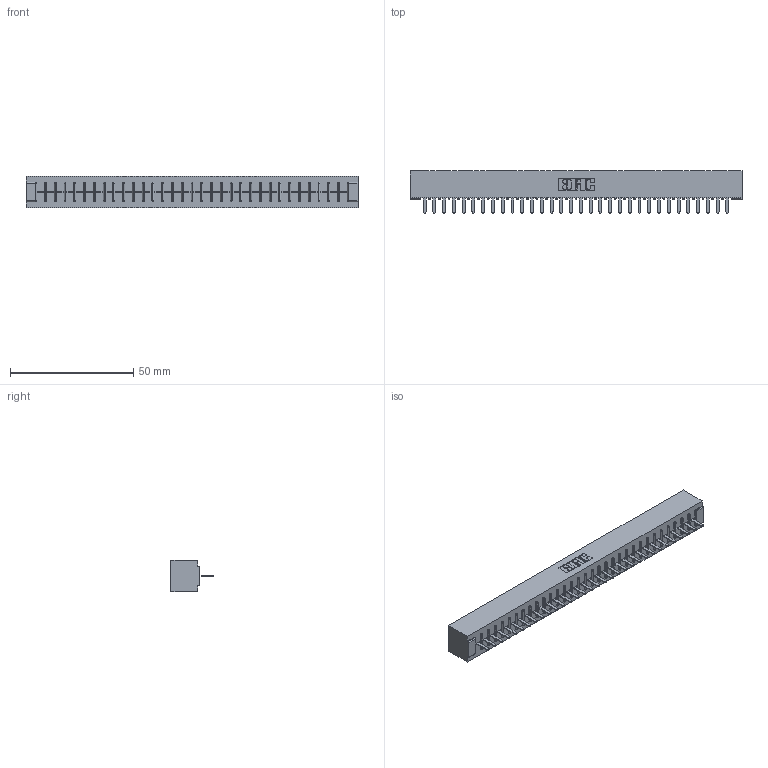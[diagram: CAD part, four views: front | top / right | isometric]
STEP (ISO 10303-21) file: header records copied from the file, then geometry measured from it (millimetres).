
FILE_DESCRIPTION (( 'STEP AP203' ), '1' );
FILE_NAME ('356-032-420-101.STEP', '2020-09-23T21:11:50', ( '' ), ( '' ), 'SwSTEP 2.0', 'SolidWorks 2020', '' );
FILE_SCHEMA (( 'CONFIG_CONTROL_DESIGN' ));
Length unit declared in the file: inch
Products named in the file (3): 306 Part_No Mounting; 306-290-001_120; 356-032-420-101
Assembly tree (33 placements, depth 2):
  356-032-420-101
    306 Part_No Mounting
    306-290-001_120  x32
Bounding box: 134.67 x 17.12 x 12.7 mm (x, y, z)
Volume: 15383.7 mm3; surface area: 15840.4 mm2
Topology: 33 solids, 33 shells, 2348 faces, 6596 edges, 4224 vertices
Faces by surface type: plane 1568, cylinder 652, sphere 128
Entity records: 30815 total; most frequent: CARTESIAN_POINT 5171, ORIENTED_EDGE 5124, DIRECTION 5100, EDGE_CURVE 2562, VECTOR 2002, LINE 2002, VERTEX_POINT 1620, AXIS2_PLACEMENT_3D 1549
